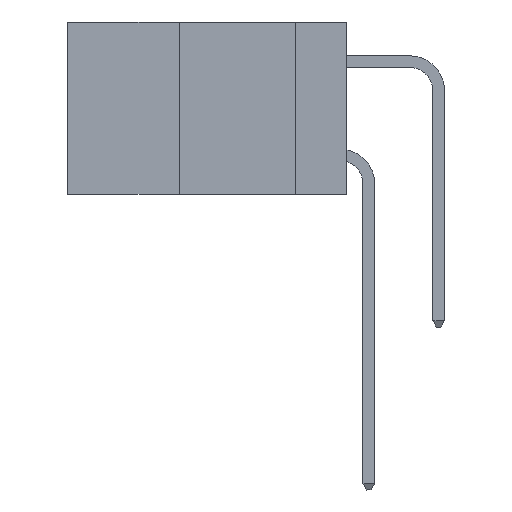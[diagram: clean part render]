
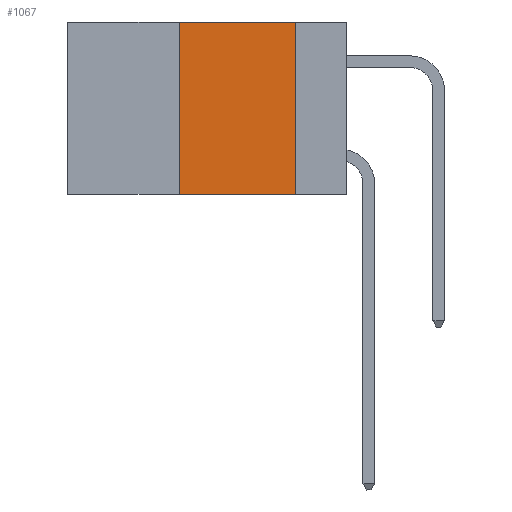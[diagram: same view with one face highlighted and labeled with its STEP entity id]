
A CAD part, left-side view. The second image highlights one B-rep face of the part: STEP entity #1067.
In plain terms, the highlighted planar face has unit normal (-1, 0, 0).
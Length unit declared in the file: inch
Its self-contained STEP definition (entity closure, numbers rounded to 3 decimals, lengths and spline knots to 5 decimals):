
#262 = EDGE_CURVE ( 'NONE', #1528, #4148, #9291, .T. ) ;
#654 = VECTOR ( 'NONE', #6486, 39.37008 ) ;
#820 = CARTESIAN_POINT ( 'NONE',  ( 0., 0.6, 0. ) ) ;
#857 = CARTESIAN_POINT ( 'NONE',  ( 0., 0.36, -0.37 ) ) ;
#875 = AXIS2_PLACEMENT_3D ( 'NONE', #820, #9910, #2353 ) ;
#1067 = ADVANCED_FACE ( 'NONE', ( #7546 ), #8968, .F. ) ;
#1528 = VERTEX_POINT ( 'NONE', #857 ) ;
#1620 = EDGE_CURVE ( 'NONE', #4148, #7183, #7551, .T. ) ;
#1749 = DIRECTION ( 'NONE',  ( 0., 0., 1. ) ) ;
#2066 = CARTESIAN_POINT ( 'NONE',  ( 0., 0.36, 0. ) ) ;
#2219 = CARTESIAN_POINT ( 'NONE',  ( 0., 0.11, -0.37 ) ) ;
#2353 = DIRECTION ( 'NONE',  ( 0., 0., -1. ) ) ;
#2548 = LINE ( 'NONE', #5746, #4466 ) ;
#2676 = CARTESIAN_POINT ( 'NONE',  ( 0., 0.6, 0. ) ) ;
#2711 = DIRECTION ( 'NONE',  ( 0., -1., 0. ) ) ;
#3102 = LINE ( 'NONE', #5682, #654 ) ;
#3139 = ORIENTED_EDGE ( 'NONE', *, *, #262, .F. ) ;
#3619 = CARTESIAN_POINT ( 'NONE',  ( 0., 0.11, 0. ) ) ;
#4148 = VERTEX_POINT ( 'NONE', #7832 ) ;
#4466 = VECTOR ( 'NONE', #6562, 39.37008 ) ;
#5349 = EDGE_LOOP ( 'NONE', ( #7406, #6602, #3139, #5547 ) ) ;
#5547 = ORIENTED_EDGE ( 'NONE', *, *, #7773, .T. ) ;
#5682 = CARTESIAN_POINT ( 'NONE',  ( 0., 0.11, 0. ) ) ;
#5746 = CARTESIAN_POINT ( 'NONE',  ( 0., 0.6, -0.37 ) ) ;
#6089 = VERTEX_POINT ( 'NONE', #2219 ) ;
#6486 = DIRECTION ( 'NONE',  ( 0., 0., -1. ) ) ;
#6562 = DIRECTION ( 'NONE',  ( 0., -1., 0. ) ) ;
#6602 = ORIENTED_EDGE ( 'NONE', *, *, #1620, .F. ) ;
#7183 = VERTEX_POINT ( 'NONE', #3619 ) ;
#7406 = ORIENTED_EDGE ( 'NONE', *, *, #7692, .F. ) ;
#7546 = FACE_OUTER_BOUND ( 'NONE', #5349, .T. ) ;
#7551 = LINE ( 'NONE', #2676, #9638 ) ;
#7692 = EDGE_CURVE ( 'NONE', #7183, #6089, #3102, .T. ) ;
#7773 = EDGE_CURVE ( 'NONE', #1528, #6089, #2548, .T. ) ;
#7832 = CARTESIAN_POINT ( 'NONE',  ( 0., 0.36, 0. ) ) ;
#8532 = VECTOR ( 'NONE', #1749, 39.37008 ) ;
#8968 = PLANE ( 'NONE',  #875 ) ;
#9291 = LINE ( 'NONE', #2066, #8532 ) ;
#9638 = VECTOR ( 'NONE', #2711, 39.37008 ) ;
#9910 = DIRECTION ( 'NONE',  ( 1., 0., 0. ) ) ;
